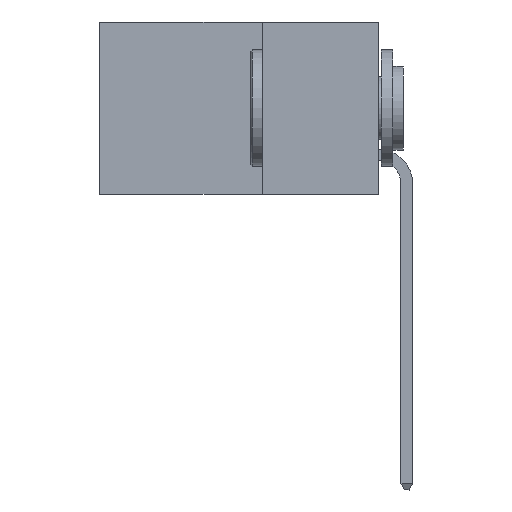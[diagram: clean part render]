
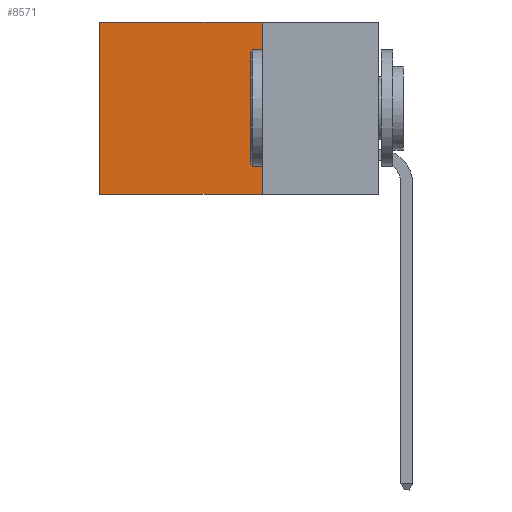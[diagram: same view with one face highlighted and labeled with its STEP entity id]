
A CAD part, left-side view. The second image highlights one B-rep face of the part: STEP entity #8571.
In plain terms, the highlighted planar face has unit normal (-1, 0, 0).
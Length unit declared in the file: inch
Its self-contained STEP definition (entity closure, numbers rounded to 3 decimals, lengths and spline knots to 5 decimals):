
#1177 = CARTESIAN_POINT ( 'NONE',  ( 0.2615, 0.25, -0.37 ) ) ;
#1471 = DIRECTION ( 'NONE',  ( 0., 1., 0. ) ) ;
#1760 = DIRECTION ( 'NONE',  ( 1., 0., 0. ) ) ;
#2893 = CARTESIAN_POINT ( 'NONE',  ( 0.2615, 0.25, 0. ) ) ;
#3451 = ORIENTED_EDGE ( 'NONE', *, *, #8175, .F. ) ;
#3754 = EDGE_CURVE ( 'NONE', #18448, #11587, #20584, .T. ) ;
#3797 = VECTOR ( 'NONE', #22163, 39.37008 ) ;
#5559 = CARTESIAN_POINT ( 'NONE',  ( 0.2615, 0.25, -0.37 ) ) ;
#8175 = EDGE_CURVE ( 'NONE', #22094, #18448, #10809, .T. ) ;
#8571 = ADVANCED_FACE ( 'NONE', ( #16448 ), #19517, .F. ) ;
#9181 = DIRECTION ( 'NONE',  ( 0., 1., 0. ) ) ;
#9789 = VECTOR ( 'NONE', #21098, 39.37008 ) ;
#10809 = LINE ( 'NONE', #1177, #3797 ) ;
#11587 = VERTEX_POINT ( 'NONE', #18292 ) ;
#11962 = CARTESIAN_POINT ( 'NONE',  ( 0.2615, 0.6, 0. ) ) ;
#12543 = VERTEX_POINT ( 'NONE', #11962 ) ;
#13803 = ORIENTED_EDGE ( 'NONE', *, *, #19007, .T. ) ;
#14535 = EDGE_LOOP ( 'NONE', ( #14866, #22258, #3451, #13803 ) ) ;
#14555 = LINE ( 'NONE', #24124, #9789 ) ;
#14866 = ORIENTED_EDGE ( 'NONE', *, *, #19813, .T. ) ;
#15257 = CARTESIAN_POINT ( 'NONE',  ( 0.2615, 0.25, 0. ) ) ;
#16448 = FACE_OUTER_BOUND ( 'NONE', #14535, .T. ) ;
#17164 = LINE ( 'NONE', #15257, #23880 ) ;
#18292 = CARTESIAN_POINT ( 'NONE',  ( 0.2615, 0.6, -0.37 ) ) ;
#18448 = VERTEX_POINT ( 'NONE', #20215 ) ;
#18759 = AXIS2_PLACEMENT_3D ( 'NONE', #5559, #1760, #22476 ) ;
#19007 = EDGE_CURVE ( 'NONE', #22094, #12543, #17164, .T. ) ;
#19517 = PLANE ( 'NONE',  #18759 ) ;
#19813 = EDGE_CURVE ( 'NONE', #12543, #11587, #14555, .T. ) ;
#20215 = CARTESIAN_POINT ( 'NONE',  ( 0.2615, 0.25, -0.37 ) ) ;
#20584 = LINE ( 'NONE', #24739, #24422 ) ;
#21098 = DIRECTION ( 'NONE',  ( 0., 0., -1. ) ) ;
#22094 = VERTEX_POINT ( 'NONE', #2893 ) ;
#22163 = DIRECTION ( 'NONE',  ( 0., 0., -1. ) ) ;
#22258 = ORIENTED_EDGE ( 'NONE', *, *, #3754, .F. ) ;
#22476 = DIRECTION ( 'NONE',  ( 0., 0., -1. ) ) ;
#23880 = VECTOR ( 'NONE', #9181, 39.37008 ) ;
#24124 = CARTESIAN_POINT ( 'NONE',  ( 0.2615, 0.6, -0.37 ) ) ;
#24422 = VECTOR ( 'NONE', #1471, 39.37008 ) ;
#24739 = CARTESIAN_POINT ( 'NONE',  ( 0.2615, 0.25, -0.37 ) ) ;
